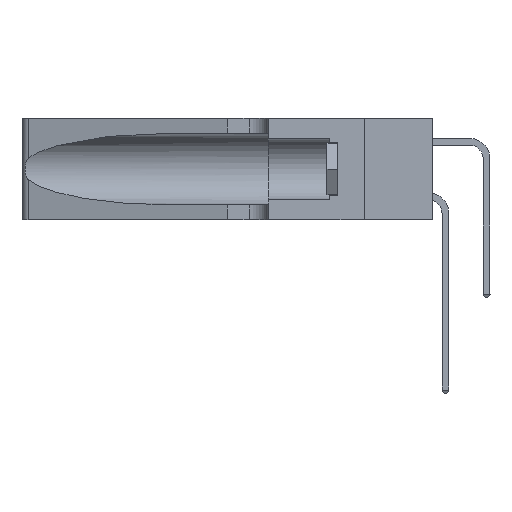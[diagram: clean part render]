
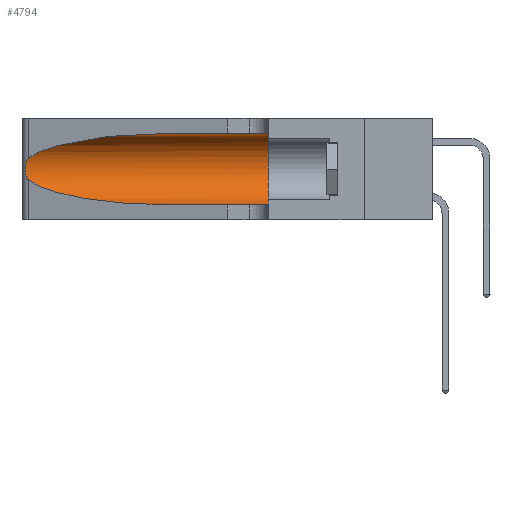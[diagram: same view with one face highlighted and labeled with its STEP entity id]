
A CAD part, left-side view. The second image highlights one B-rep face of the part: STEP entity #4794.
In plain terms, the highlighted cylindrical face has radius 3.308 mm (diameter 6.617 mm), a partial arc.
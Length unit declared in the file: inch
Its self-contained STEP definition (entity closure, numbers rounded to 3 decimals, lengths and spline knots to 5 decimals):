
#569 = EDGE_CURVE ( 'NONE', #5403, #4991, #9108, .T. ) ;
#1716 = CARTESIAN_POINT ( 'NONE',  ( 0.1305, 1.61858, 0.185 ) ) ;
#1761 = CARTESIAN_POINT ( 'NONE',  ( 0.25854, 1.2359, 0.20912 ) ) ;
#1764 = CARTESIAN_POINT ( 'NONE',  ( 0.1305, 1.61858, 0.05475 ) ) ;
#1850 = CARTESIAN_POINT ( 'NONE',  ( 0.1305, 0.35, 0.185 ) ) ;
#1935 = CARTESIAN_POINT ( 'NONE',  ( 0.25787, 1.23484, 0.2124 ) ) ;
#2111 = LINE ( 'NONE', #1764, #6795 ) ;
#3473 = ORIENTED_EDGE ( 'NONE', *, *, #9117, .F. ) ;
#3605 = CARTESIAN_POINT ( 'NONE',  ( 0.1305, 0.72297, 0.31525 ) ) ;
#3742 = CARTESIAN_POINT ( 'NONE',  ( 0.26018, 1.23835, 0.19895 ) ) ;
#3908 = CARTESIAN_POINT ( 'NONE',  ( 0.1305, 0.72297, 0.05475 ) ) ;
#4254 = CARTESIAN_POINT ( 'NONE',  ( 0.25856, 1.23593, 0.16098 ) ) ;
#4260 = CARTESIAN_POINT ( 'NONE',  ( 0.1305, 0.72297, 0.31525 ) ) ;
#4483 = ORIENTED_EDGE ( 'NONE', *, *, #16032, .T. ) ;
#4519 = CARTESIAN_POINT ( 'NONE',  ( 0.25789, 1.23486, 0.15765 ) ) ;
#4794 = ADVANCED_FACE ( 'NONE', ( #25099 ), #23860, .F. ) ;
#4808 = VERTEX_POINT ( 'NONE', #11470 ) ;
#4991 = VERTEX_POINT ( 'NONE', #10231 ) ;
#5403 = VERTEX_POINT ( 'NONE', #4260 ) ;
#5650 = ORIENTED_EDGE ( 'NONE', *, *, #5825, .T. ) ;
#5825 = EDGE_CURVE ( 'NONE', #19685, #19629, #16050, .T. ) ;
#6551 = CARTESIAN_POINT ( 'NONE',  ( 0.25487, 1.22718, 0.14631 ) ) ;
#6795 = VECTOR ( 'NONE', #19858, 39.37008 ) ;
#6806 = AXIS2_PLACEMENT_3D ( 'NONE', #1850, #21768, #10249 ) ;
#6849 =( BOUNDED_CURVE ( )  B_SPLINE_CURVE ( 3, ( #9945, #16075, #7939, #3908 ),
 .UNSPECIFIED., .F., .T. ) 
 B_SPLINE_CURVE_WITH_KNOTS ( ( 4, 4 ),
 ( 3.44316, 4.71239 ),
 .UNSPECIFIED. ) 
 CURVE ( )  GEOMETRIC_REPRESENTATION_ITEM ( )  RATIONAL_B_SPLINE_CURVE ( ( 1., 0.87, 0.87, 1. ) ) 
 REPRESENTATION_ITEM ( '' )  );
#7542 = EDGE_LOOP ( 'NONE', ( #4483, #5650, #21250, #11216, #3473, #13471 ) ) ;
#7939 = CARTESIAN_POINT ( 'NONE',  ( 0.18966, 0.96281, 0.05475 ) ) ;
#8377 = CARTESIAN_POINT ( 'NONE',  ( 0.26075, 1.23896, 0.19203 ) ) ;
#8522 = CARTESIAN_POINT ( 'NONE',  ( 0.1305, 1.61858, 0.31525 ) ) ;
#9108 = LINE ( 'NONE', #8522, #13130 ) ;
#9117 = EDGE_CURVE ( 'NONE', #4991, #4808, #20459, .T. ) ;
#9243 = VERTEX_POINT ( 'NONE', #23409 ) ;
#9945 = CARTESIAN_POINT ( 'NONE',  ( 0.25487, 1.22718, 0.14631 ) ) ;
#10231 = CARTESIAN_POINT ( 'NONE',  ( 0.1305, 0.35, 0.31525 ) ) ;
#10249 = DIRECTION ( 'NONE',  ( 0., 0., 1. ) ) ;
#11216 = ORIENTED_EDGE ( 'NONE', *, *, #24197, .T. ) ;
#11470 = CARTESIAN_POINT ( 'NONE',  ( 0.1305, 0.35, 0.05475 ) ) ;
#12115 = CARTESIAN_POINT ( 'NONE',  ( 0.25639, 1.23186, 0.15144 ) ) ;
#13130 = VECTOR ( 'NONE', #22501, 39.37008 ) ;
#13471 = ORIENTED_EDGE ( 'NONE', *, *, #569, .F. ) ;
#13656 = CARTESIAN_POINT ( 'NONE',  ( 0.25639, 1.23184, 0.21858 ) ) ;
#14335 = CARTESIAN_POINT ( 'NONE',  ( 0.26075, 1.23896, 0.178 ) ) ;
#15796 = DIRECTION ( 'NONE',  ( 0., 0., -1. ) ) ;
#16032 = EDGE_CURVE ( 'NONE', #5403, #19685, #19578, .T. ) ;
#16050 = B_SPLINE_CURVE_WITH_KNOTS ( 'NONE', 3,
 ( #20029, #23582, #13656, #1935, #1761, #3742, #8377, #14335, #16320, #4254, #4519, #12115, #18180, #6551 ),
 .UNSPECIFIED., .F., .F.,
 ( 4, 2, 2, 2, 2, 2, 4 ),
 ( 0., 0.00027, 0.00053, 0.00107, 0.0016, 0.00187, 0.00214 ),
 .UNSPECIFIED. ) ;
#16075 = CARTESIAN_POINT ( 'NONE',  ( 0.2373, 1.15595, 0.08982 ) ) ;
#16320 = CARTESIAN_POINT ( 'NONE',  ( 0.26017, 1.23833, 0.17102 ) ) ;
#16870 = CARTESIAN_POINT ( 'NONE',  ( 0.25487, 1.22718, 0.14631 ) ) ;
#17591 = DIRECTION ( 'NONE',  ( 0., -1., 0. ) ) ;
#18180 = CARTESIAN_POINT ( 'NONE',  ( 0.25555, 1.22993, 0.14849 ) ) ;
#19448 = CARTESIAN_POINT ( 'NONE',  ( 0.18966, 0.96281, 0.31525 ) ) ;
#19578 =( BOUNDED_CURVE ( )  B_SPLINE_CURVE ( 3, ( #3605, #19448, #21548, #25191 ),
 .UNSPECIFIED., .F., .F. ) 
 B_SPLINE_CURVE_WITH_KNOTS ( ( 4, 4 ),
 ( 1.5708, 2.84003 ),
 .UNSPECIFIED. ) 
 CURVE ( )  GEOMETRIC_REPRESENTATION_ITEM ( )  RATIONAL_B_SPLINE_CURVE ( ( 1., 0.87, 0.87, 1. ) ) 
 REPRESENTATION_ITEM ( '' )  );
#19629 = VERTEX_POINT ( 'NONE', #16870 ) ;
#19685 = VERTEX_POINT ( 'NONE', #22989 ) ;
#19858 = DIRECTION ( 'NONE',  ( 0., -1., 0. ) ) ;
#20029 = CARTESIAN_POINT ( 'NONE',  ( 0.25487, 1.22718, 0.22369 ) ) ;
#20459 = CIRCLE ( 'NONE', #6806, 0.13025 ) ;
#21250 = ORIENTED_EDGE ( 'NONE', *, *, #22991, .T. ) ;
#21548 = CARTESIAN_POINT ( 'NONE',  ( 0.2373, 1.15595, 0.28018 ) ) ;
#21768 = DIRECTION ( 'NONE',  ( 0., 1., 0. ) ) ;
#22501 = DIRECTION ( 'NONE',  ( 0., -1., 0. ) ) ;
#22989 = CARTESIAN_POINT ( 'NONE',  ( 0.25487, 1.22718, 0.22369 ) ) ;
#22991 = EDGE_CURVE ( 'NONE', #19629, #9243, #6849, .T. ) ;
#23393 = AXIS2_PLACEMENT_3D ( 'NONE', #1716, #17591, #15796 ) ;
#23409 = CARTESIAN_POINT ( 'NONE',  ( 0.1305, 0.72297, 0.05475 ) ) ;
#23582 = CARTESIAN_POINT ( 'NONE',  ( 0.25555, 1.22994, 0.2215 ) ) ;
#23860 = CYLINDRICAL_SURFACE ( 'NONE', #23393, 0.13025 ) ;
#24197 = EDGE_CURVE ( 'NONE', #9243, #4808, #2111, .T. ) ;
#25099 = FACE_OUTER_BOUND ( 'NONE', #7542, .T. ) ;
#25191 = CARTESIAN_POINT ( 'NONE',  ( 0.25487, 1.22718, 0.22369 ) ) ;
